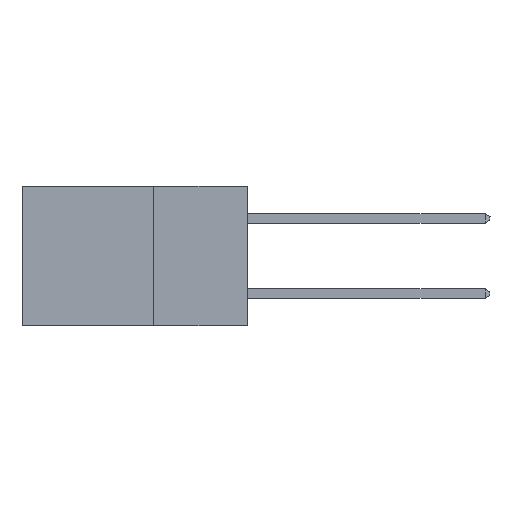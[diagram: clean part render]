
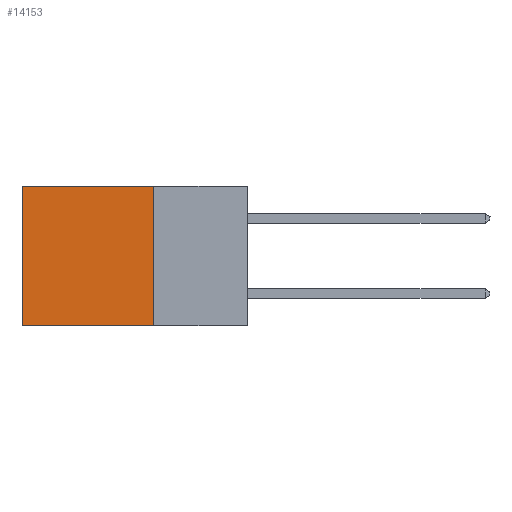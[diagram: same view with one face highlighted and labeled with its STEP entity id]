
A CAD part, left-side view. The second image highlights one B-rep face of the part: STEP entity #14153.
In plain terms, the highlighted planar face has unit normal (-1, 0, 0).
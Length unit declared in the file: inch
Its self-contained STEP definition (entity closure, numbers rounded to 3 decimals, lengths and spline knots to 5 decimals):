
#2046 = CARTESIAN_POINT ( 'NONE',  ( 0.2615, 0.6, 0. ) ) ;
#2485 = ORIENTED_EDGE ( 'NONE', *, *, #5456, .F. ) ;
#3259 = FACE_OUTER_BOUND ( 'NONE', #15898, .T. ) ;
#3603 = VECTOR ( 'NONE', #7345, 39.37008 ) ;
#3607 = ORIENTED_EDGE ( 'NONE', *, *, #13264, .T. ) ;
#3803 = DIRECTION ( 'NONE',  ( 0., 1., 0. ) ) ;
#4175 = VERTEX_POINT ( 'NONE', #11899 ) ;
#4218 = ORIENTED_EDGE ( 'NONE', *, *, #14679, .T. ) ;
#4418 = VECTOR ( 'NONE', #12602, 39.37008 ) ;
#4584 = CARTESIAN_POINT ( 'NONE',  ( 0.2615, 0.25, -0.37 ) ) ;
#4667 = VERTEX_POINT ( 'NONE', #2046 ) ;
#5456 = EDGE_CURVE ( 'NONE', #4175, #13039, #15406, .T. ) ;
#5976 = DIRECTION ( 'NONE',  ( 1., 0., 0. ) ) ;
#7105 = PLANE ( 'NONE',  #7766 ) ;
#7192 = EDGE_CURVE ( 'NONE', #13039, #9053, #17323, .T. ) ;
#7345 = DIRECTION ( 'NONE',  ( 0., 0., -1. ) ) ;
#7766 = AXIS2_PLACEMENT_3D ( 'NONE', #4584, #5976, #15262 ) ;
#8053 = VECTOR ( 'NONE', #16647, 39.37008 ) ;
#8177 = LINE ( 'NONE', #13591, #4418 ) ;
#8883 = CARTESIAN_POINT ( 'NONE',  ( 0.2615, 0.25, -0.37 ) ) ;
#9053 = VERTEX_POINT ( 'NONE', #10505 ) ;
#10079 = CARTESIAN_POINT ( 'NONE',  ( 0.2615, 0.25, 0. ) ) ;
#10505 = CARTESIAN_POINT ( 'NONE',  ( 0.2615, 0.6, -0.37 ) ) ;
#11232 = CARTESIAN_POINT ( 'NONE',  ( 0.2615, 0.25, -0.37 ) ) ;
#11456 = CARTESIAN_POINT ( 'NONE',  ( 0.2615, 0.25, -0.37 ) ) ;
#11899 = CARTESIAN_POINT ( 'NONE',  ( 0.2615, 0.25, 0. ) ) ;
#12602 = DIRECTION ( 'NONE',  ( 0., 0., -1. ) ) ;
#13039 = VERTEX_POINT ( 'NONE', #11456 ) ;
#13264 = EDGE_CURVE ( 'NONE', #4175, #4667, #13865, .T. ) ;
#13566 = ORIENTED_EDGE ( 'NONE', *, *, #7192, .F. ) ;
#13591 = CARTESIAN_POINT ( 'NONE',  ( 0.2615, 0.6, -0.37 ) ) ;
#13865 = LINE ( 'NONE', #10079, #8053 ) ;
#14153 = ADVANCED_FACE ( 'NONE', ( #3259 ), #7105, .F. ) ;
#14679 = EDGE_CURVE ( 'NONE', #4667, #9053, #8177, .T. ) ;
#15262 = DIRECTION ( 'NONE',  ( 0., 0., -1. ) ) ;
#15406 = LINE ( 'NONE', #11232, #3603 ) ;
#15898 = EDGE_LOOP ( 'NONE', ( #4218, #13566, #2485, #3607 ) ) ;
#16201 = VECTOR ( 'NONE', #3803, 39.37008 ) ;
#16647 = DIRECTION ( 'NONE',  ( 0., 1., 0. ) ) ;
#17323 = LINE ( 'NONE', #8883, #16201 ) ;
